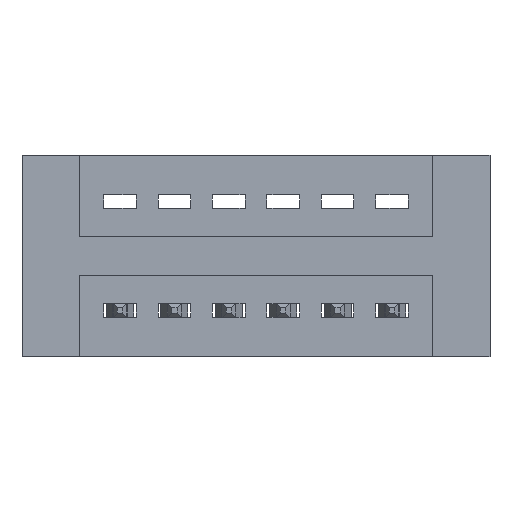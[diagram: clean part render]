
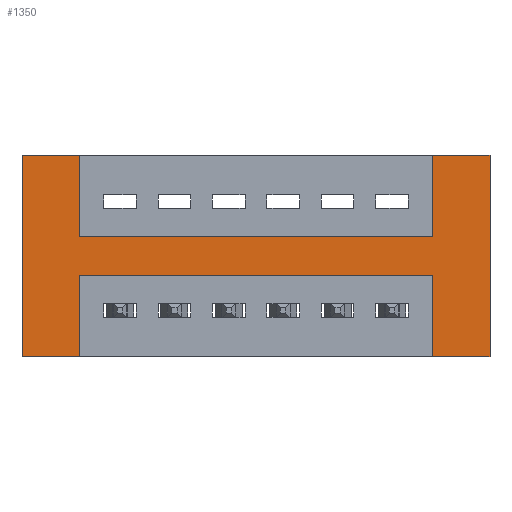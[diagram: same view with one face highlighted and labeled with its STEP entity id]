
A CAD part, front view. The second image highlights one B-rep face of the part: STEP entity #1350.
In plain terms, the highlighted planar face has unit normal (0, -1, 0).
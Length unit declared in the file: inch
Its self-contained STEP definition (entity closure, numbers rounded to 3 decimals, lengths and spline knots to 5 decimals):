
#81 = VECTOR ( 'NONE', #315, 39.37008 ) ;
#103 = VERTEX_POINT ( 'NONE', #1049 ) ;
#194 = CARTESIAN_POINT ( 'NONE',  ( 1.1475, 0., -0.37 ) ) ;
#315 = DIRECTION ( 'NONE',  ( 0., 0., 1. ) ) ;
#340 = CARTESIAN_POINT ( 'NONE',  ( 0.3925, 0., -0.22 ) ) ;
#350 = CARTESIAN_POINT ( 'NONE',  ( 1.0425, 0., 0. ) ) ;
#382 = CARTESIAN_POINT ( 'NONE',  ( 0., 0., 0. ) ) ;
#434 = DIRECTION ( 'NONE',  ( 1., 0., 0. ) ) ;
#476 = LINE ( 'NONE', #6644, #6427 ) ;
#531 = VERTEX_POINT ( 'NONE', #6539 ) ;
#585 = DIRECTION ( 'NONE',  ( -1., 0., 0. ) ) ;
#679 = VERTEX_POINT ( 'NONE', #4993 ) ;
#730 = DIRECTION ( 'NONE',  ( 0., 0., -1. ) ) ;
#865 = VECTOR ( 'NONE', #4283, 39.37008 ) ;
#1023 = CARTESIAN_POINT ( 'NONE',  ( 0.3925, 0., 0. ) ) ;
#1049 = CARTESIAN_POINT ( 'NONE',  ( 0.2875, 0., 0. ) ) ;
#1142 = CARTESIAN_POINT ( 'NONE',  ( 0.3925, 0., -0.22 ) ) ;
#1282 = CARTESIAN_POINT ( 'NONE',  ( 0., 0., -0.37 ) ) ;
#1287 = EDGE_CURVE ( 'NONE', #2534, #4313, #8712, .T. ) ;
#1307 = DIRECTION ( 'NONE',  ( 0., 0., -1. ) ) ;
#1350 = ADVANCED_FACE ( 'NONE', ( #2728 ), #1414, .T. ) ;
#1359 = VECTOR ( 'NONE', #434, 39.37008 ) ;
#1414 = PLANE ( 'NONE',  #1538 ) ;
#1455 = DIRECTION ( 'NONE',  ( 0., -1., 0. ) ) ;
#1467 = CARTESIAN_POINT ( 'NONE',  ( 0.3925, 0., -0.37 ) ) ;
#1494 = DIRECTION ( 'NONE',  ( 0., 0., -1. ) ) ;
#1538 = AXIS2_PLACEMENT_3D ( 'NONE', #1282, #1455, #1494 ) ;
#1610 = DIRECTION ( 'NONE',  ( 0., 0., 1. ) ) ;
#1784 = CARTESIAN_POINT ( 'NONE',  ( 1.0425, 0., -0.37 ) ) ;
#2193 = CARTESIAN_POINT ( 'NONE',  ( 0., 0., -0.37 ) ) ;
#2387 = DIRECTION ( 'NONE',  ( 0., 0., -1. ) ) ;
#2402 = LINE ( 'NONE', #5922, #5954 ) ;
#2452 = CARTESIAN_POINT ( 'NONE',  ( 0., 0., 0. ) ) ;
#2487 = VERTEX_POINT ( 'NONE', #4623 ) ;
#2534 = VERTEX_POINT ( 'NONE', #5907 ) ;
#2566 = CARTESIAN_POINT ( 'NONE',  ( 1.0425, 0., -0.22 ) ) ;
#2570 = ORIENTED_EDGE ( 'NONE', *, *, #4770, .F. ) ;
#2638 = EDGE_CURVE ( 'NONE', #531, #2487, #6679, .T. ) ;
#2728 = FACE_OUTER_BOUND ( 'NONE', #8732, .T. ) ;
#2860 = VECTOR ( 'NONE', #6311, 39.37008 ) ;
#3221 = CARTESIAN_POINT ( 'NONE',  ( 1.1475, 0., 0. ) ) ;
#3538 = VECTOR ( 'NONE', #8552, 39.37008 ) ;
#3728 = ORIENTED_EDGE ( 'NONE', *, *, #7530, .F. ) ;
#3945 = EDGE_CURVE ( 'NONE', #2487, #5304, #476, .T. ) ;
#3970 = LINE ( 'NONE', #2452, #3538 ) ;
#4179 = EDGE_CURVE ( 'NONE', #103, #5975, #5092, .T. ) ;
#4283 = DIRECTION ( 'NONE',  ( -1., 0., 0. ) ) ;
#4299 = EDGE_CURVE ( 'NONE', #5304, #2534, #7663, .T. ) ;
#4313 = VERTEX_POINT ( 'NONE', #3221 ) ;
#4553 = CARTESIAN_POINT ( 'NONE',  ( 1.0425, 0., -0.15 ) ) ;
#4607 = ORIENTED_EDGE ( 'NONE', *, *, #5491, .F. ) ;
#4623 = CARTESIAN_POINT ( 'NONE',  ( 0.3925, 0., -0.15 ) ) ;
#4675 = EDGE_CURVE ( 'NONE', #679, #8947, #5081, .T. ) ;
#4770 = EDGE_CURVE ( 'NONE', #9120, #5800, #6308, .T. ) ;
#4853 = LINE ( 'NONE', #2193, #865 ) ;
#4893 = DIRECTION ( 'NONE',  ( 1., 0., 0. ) ) ;
#4993 = CARTESIAN_POINT ( 'NONE',  ( 1.0425, 0., -0.37 ) ) ;
#5081 = LINE ( 'NONE', #1784, #6751 ) ;
#5092 = LINE ( 'NONE', #7291, #8400 ) ;
#5174 = ORIENTED_EDGE ( 'NONE', *, *, #5186, .F. ) ;
#5176 = LINE ( 'NONE', #6334, #2860 ) ;
#5186 = EDGE_CURVE ( 'NONE', #5800, #5975, #4853, .T. ) ;
#5304 = VERTEX_POINT ( 'NONE', #4553 ) ;
#5376 = ORIENTED_EDGE ( 'NONE', *, *, #1287, .F. ) ;
#5408 = ORIENTED_EDGE ( 'NONE', *, *, #4299, .F. ) ;
#5491 = EDGE_CURVE ( 'NONE', #8947, #9120, #7537, .T. ) ;
#5552 = VERTEX_POINT ( 'NONE', #194 ) ;
#5800 = VERTEX_POINT ( 'NONE', #6969 ) ;
#5811 = CARTESIAN_POINT ( 'NONE',  ( 0.2875, 0., -0.37 ) ) ;
#5877 = EDGE_CURVE ( 'NONE', #5552, #4313, #5176, .T. ) ;
#5907 = CARTESIAN_POINT ( 'NONE',  ( 1.0425, 0., 0. ) ) ;
#5922 = CARTESIAN_POINT ( 'NONE',  ( 0., 0., -0.37 ) ) ;
#5954 = VECTOR ( 'NONE', #6005, 39.37008 ) ;
#5964 = EDGE_CURVE ( 'NONE', #5552, #679, #2402, .T. ) ;
#5975 = VERTEX_POINT ( 'NONE', #5811 ) ;
#6005 = DIRECTION ( 'NONE',  ( -1., 0., 0. ) ) ;
#6129 = ORIENTED_EDGE ( 'NONE', *, *, #5877, .T. ) ;
#6308 = LINE ( 'NONE', #1467, #8056 ) ;
#6311 = DIRECTION ( 'NONE',  ( 0., 0., 1. ) ) ;
#6334 = CARTESIAN_POINT ( 'NONE',  ( 1.1475, 0., 0. ) ) ;
#6365 = ORIENTED_EDGE ( 'NONE', *, *, #2638, .F. ) ;
#6427 = VECTOR ( 'NONE', #4893, 39.37008 ) ;
#6539 = CARTESIAN_POINT ( 'NONE',  ( 0.3925, 0., 0. ) ) ;
#6644 = CARTESIAN_POINT ( 'NONE',  ( 0.3925, 0., -0.15 ) ) ;
#6679 = LINE ( 'NONE', #1023, #8339 ) ;
#6726 = ORIENTED_EDGE ( 'NONE', *, *, #4675, .F. ) ;
#6751 = VECTOR ( 'NONE', #1610, 39.37008 ) ;
#6817 = ORIENTED_EDGE ( 'NONE', *, *, #3945, .F. ) ;
#6969 = CARTESIAN_POINT ( 'NONE',  ( 0.3925, 0., -0.37 ) ) ;
#7046 = ORIENTED_EDGE ( 'NONE', *, *, #4179, .T. ) ;
#7291 = CARTESIAN_POINT ( 'NONE',  ( 0.2875, 0., 0. ) ) ;
#7488 = ORIENTED_EDGE ( 'NONE', *, *, #5964, .F. ) ;
#7530 = EDGE_CURVE ( 'NONE', #103, #531, #3970, .T. ) ;
#7537 = LINE ( 'NONE', #340, #7958 ) ;
#7663 = LINE ( 'NONE', #350, #81 ) ;
#7958 = VECTOR ( 'NONE', #585, 39.37008 ) ;
#8056 = VECTOR ( 'NONE', #1307, 39.37008 ) ;
#8339 = VECTOR ( 'NONE', #730, 39.37008 ) ;
#8400 = VECTOR ( 'NONE', #2387, 39.37008 ) ;
#8552 = DIRECTION ( 'NONE',  ( 1., 0., 0. ) ) ;
#8712 = LINE ( 'NONE', #382, #1359 ) ;
#8732 = EDGE_LOOP ( 'NONE', ( #6129, #5376, #5408, #6817, #6365, #3728, #7046, #5174, #2570, #4607, #6726, #7488 ) ) ;
#8947 = VERTEX_POINT ( 'NONE', #2566 ) ;
#9120 = VERTEX_POINT ( 'NONE', #1142 ) ;
